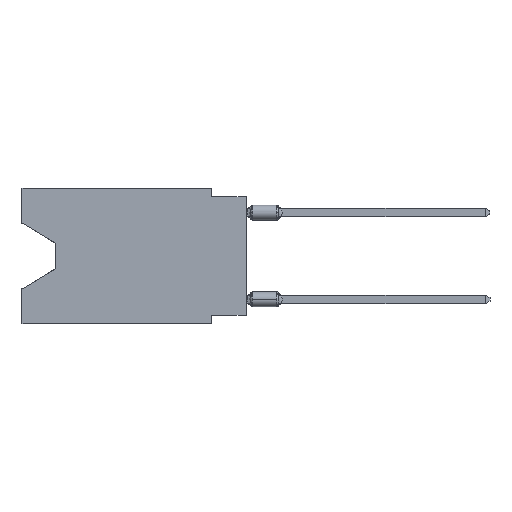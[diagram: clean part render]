
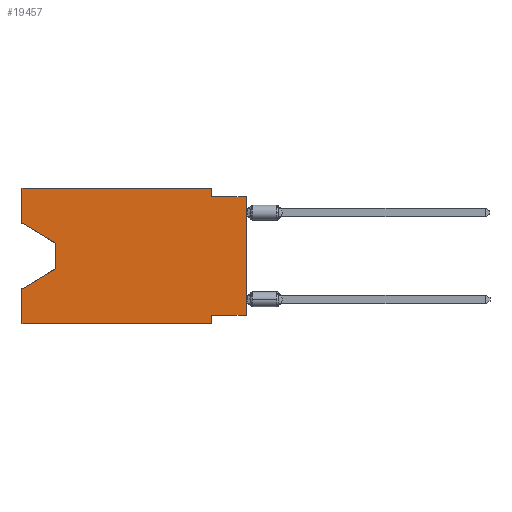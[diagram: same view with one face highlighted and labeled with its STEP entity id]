
A CAD part, left-side view. The second image highlights one B-rep face of the part: STEP entity #19457.
In plain terms, the highlighted planar face has unit normal (-1, 0, 0).
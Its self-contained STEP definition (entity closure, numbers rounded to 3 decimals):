
#6 = ORIENTED_EDGE ( 'NONE', *, *, #12105, .T. ) ;
#23 = DIRECTION ( 'NONE',  ( 0., 0., 1. ) ) ;
#48 = DIRECTION ( 'NONE',  ( 1., 0., 0. ) ) ;
#96 = VERTEX_POINT ( 'NONE', #19820 ) ;
#188 = VERTEX_POINT ( 'NONE', #5122 ) ;
#395 = EDGE_CURVE ( 'NONE', #18497, #10183, #13707, .T. ) ;
#410 = EDGE_CURVE ( 'NONE', #188, #12576, #13610, .T. ) ;
#432 = ORIENTED_EDGE ( 'NONE', *, *, #410, .F. ) ;
#575 = VECTOR ( 'NONE', #6112, 1000. ) ;
#584 = DIRECTION ( 'NONE',  ( 0., 0., -1. ) ) ;
#1484 = EDGE_CURVE ( 'NONE', #18497, #5550, #7047, .T. ) ;
#2035 = ORIENTED_EDGE ( 'NONE', *, *, #1484, .F. ) ;
#2801 = LINE ( 'NONE', #13636, #12049 ) ;
#2928 = ORIENTED_EDGE ( 'NONE', *, *, #8301, .F. ) ;
#3142 = LINE ( 'NONE', #4564, #7276 ) ;
#3235 = EDGE_CURVE ( 'NONE', #8358, #5016, #3142, .T. ) ;
#3303 = CARTESIAN_POINT ( 'NONE',  ( 0., 16.383, -7.36 ) ) ;
#3586 = ORIENTED_EDGE ( 'NONE', *, *, #6259, .T. ) ;
#3788 = LINE ( 'NONE', #9570, #3892 ) ;
#3892 = VECTOR ( 'NONE', #9961, 1000. ) ;
#4329 = CARTESIAN_POINT ( 'NONE',  ( 0., 0., -9.271 ) ) ;
#4336 = DIRECTION ( 'NONE',  ( 0., -1., 0. ) ) ;
#4409 = EDGE_CURVE ( 'NONE', #13346, #12576, #11867, .T. ) ;
#4564 = CARTESIAN_POINT ( 'NONE',  ( 0., 16.383, -9.906 ) ) ;
#4571 = EDGE_CURVE ( 'NONE', #8358, #17989, #9231, .T. ) ;
#4595 = DIRECTION ( 'NONE',  ( 0., 0., -1. ) ) ;
#4759 = DIRECTION ( 'NONE',  ( 0., 0., -1. ) ) ;
#4865 = LINE ( 'NONE', #5981, #16042 ) ;
#4895 = CARTESIAN_POINT ( 'NONE',  ( 0., 16.383, 0. ) ) ;
#5016 = VERTEX_POINT ( 'NONE', #13653 ) ;
#5122 = CARTESIAN_POINT ( 'NONE',  ( 0., 2.54, -0.635 ) ) ;
#5550 = VERTEX_POINT ( 'NONE', #9500 ) ;
#5941 = LINE ( 'NONE', #12120, #8393 ) ;
#5981 = CARTESIAN_POINT ( 'NONE',  ( 0., 13.97, -4.013 ) ) ;
#6110 = AXIS2_PLACEMENT_3D ( 'NONE', #4895, #48, #4595 ) ;
#6112 = DIRECTION ( 'NONE',  ( 0., -0.855, -0.519 ) ) ;
#6210 = PLANE ( 'NONE',  #6110 ) ;
#6259 = EDGE_CURVE ( 'NONE', #10183, #96, #4865, .T. ) ;
#6454 = VECTOR ( 'NONE', #8933, 1000. ) ;
#7047 = LINE ( 'NONE', #13221, #9094 ) ;
#7091 = CARTESIAN_POINT ( 'NONE',  ( 0., 13.97, -5.893 ) ) ;
#7268 = VECTOR ( 'NONE', #10133, 1000. ) ;
#7276 = VECTOR ( 'NONE', #15584, 1000. ) ;
#7701 = CARTESIAN_POINT ( 'NONE',  ( 0., 16.383, 0. ) ) ;
#7963 = EDGE_LOOP ( 'NONE', ( #16081, #3586, #6, #18098, #18422, #8142, #2928, #16766, #432, #14068, #9190, #2035 ) ) ;
#8142 = ORIENTED_EDGE ( 'NONE', *, *, #13563, .F. ) ;
#8213 = VERTEX_POINT ( 'NONE', #12510 ) ;
#8301 = EDGE_CURVE ( 'NONE', #13346, #8213, #2801, .T. ) ;
#8358 = VERTEX_POINT ( 'NONE', #17166 ) ;
#8393 = VECTOR ( 'NONE', #584, 1000. ) ;
#8933 = DIRECTION ( 'NONE',  ( 0., 0., 1. ) ) ;
#9094 = VECTOR ( 'NONE', #19455, 1000. ) ;
#9190 = ORIENTED_EDGE ( 'NONE', *, *, #15755, .F. ) ;
#9231 = LINE ( 'NONE', #7701, #17757 ) ;
#9277 = VERTEX_POINT ( 'NONE', #14290 ) ;
#9500 = CARTESIAN_POINT ( 'NONE',  ( 0., 16.383, 0. ) ) ;
#9570 = CARTESIAN_POINT ( 'NONE',  ( 0., 2.54, 0. ) ) ;
#9961 = DIRECTION ( 'NONE',  ( 0., 0., -1. ) ) ;
#10133 = DIRECTION ( 'NONE',  ( 0., 0.855, -0.519 ) ) ;
#10183 = VERTEX_POINT ( 'NONE', #16934 ) ;
#10544 = CARTESIAN_POINT ( 'NONE',  ( 0., 0., 0. ) ) ;
#10964 = FACE_OUTER_BOUND ( 'NONE', #7963, .T. ) ;
#11867 = LINE ( 'NONE', #10544, #6454 ) ;
#12049 = VECTOR ( 'NONE', #15439, 1000. ) ;
#12105 = EDGE_CURVE ( 'NONE', #96, #17989, #17822, .T. ) ;
#12119 = CARTESIAN_POINT ( 'NONE',  ( 0., 0., -0.635 ) ) ;
#12120 = CARTESIAN_POINT ( 'NONE',  ( 0., 2.54, -9.906 ) ) ;
#12389 = DIRECTION ( 'NONE',  ( 0., -1., 0. ) ) ;
#12510 = CARTESIAN_POINT ( 'NONE',  ( 0., 2.54, -9.271 ) ) ;
#12576 = VERTEX_POINT ( 'NONE', #12119 ) ;
#13221 = CARTESIAN_POINT ( 'NONE',  ( 0., 16.383, 0. ) ) ;
#13346 = VERTEX_POINT ( 'NONE', #4329 ) ;
#13563 = EDGE_CURVE ( 'NONE', #8213, #5016, #5941, .T. ) ;
#13610 = LINE ( 'NONE', #15316, #15102 ) ;
#13636 = CARTESIAN_POINT ( 'NONE',  ( 0., 0., -9.271 ) ) ;
#13644 = CARTESIAN_POINT ( 'NONE',  ( 0., 16.383, 0. ) ) ;
#13653 = CARTESIAN_POINT ( 'NONE',  ( 0., 2.54, -9.906 ) ) ;
#13707 = LINE ( 'NONE', #19768, #575 ) ;
#14068 = ORIENTED_EDGE ( 'NONE', *, *, #16326, .F. ) ;
#14290 = CARTESIAN_POINT ( 'NONE',  ( 0., 2.54, 0. ) ) ;
#14532 = VECTOR ( 'NONE', #4336, 1000. ) ;
#15102 = VECTOR ( 'NONE', #12389, 1000. ) ;
#15316 = CARTESIAN_POINT ( 'NONE',  ( 0., 0., -0.635 ) ) ;
#15439 = DIRECTION ( 'NONE',  ( 0., 1., 0. ) ) ;
#15584 = DIRECTION ( 'NONE',  ( 0., -1., 0. ) ) ;
#15755 = EDGE_CURVE ( 'NONE', #5550, #9277, #16371, .T. ) ;
#16042 = VECTOR ( 'NONE', #4759, 1000. ) ;
#16081 = ORIENTED_EDGE ( 'NONE', *, *, #395, .T. ) ;
#16326 = EDGE_CURVE ( 'NONE', #9277, #188, #3788, .T. ) ;
#16371 = LINE ( 'NONE', #13644, #14532 ) ;
#16766 = ORIENTED_EDGE ( 'NONE', *, *, #4409, .T. ) ;
#16934 = CARTESIAN_POINT ( 'NONE',  ( 0., 13.97, -4.013 ) ) ;
#17166 = CARTESIAN_POINT ( 'NONE',  ( 0., 16.383, -9.906 ) ) ;
#17757 = VECTOR ( 'NONE', #23, 1000. ) ;
#17822 = LINE ( 'NONE', #7091, #7268 ) ;
#17989 = VERTEX_POINT ( 'NONE', #3303 ) ;
#18098 = ORIENTED_EDGE ( 'NONE', *, *, #4571, .F. ) ;
#18422 = ORIENTED_EDGE ( 'NONE', *, *, #3235, .T. ) ;
#18497 = VERTEX_POINT ( 'NONE', #18952 ) ;
#18952 = CARTESIAN_POINT ( 'NONE',  ( 0., 16.383, -2.546 ) ) ;
#19455 = DIRECTION ( 'NONE',  ( 0., 0., 1. ) ) ;
#19457 = ADVANCED_FACE ( 'NONE', ( #10964 ), #6210, .F. ) ;
#19768 = CARTESIAN_POINT ( 'NONE',  ( 0., 16.383, -2.546 ) ) ;
#19820 = CARTESIAN_POINT ( 'NONE',  ( 0., 13.97, -5.893 ) ) ;
